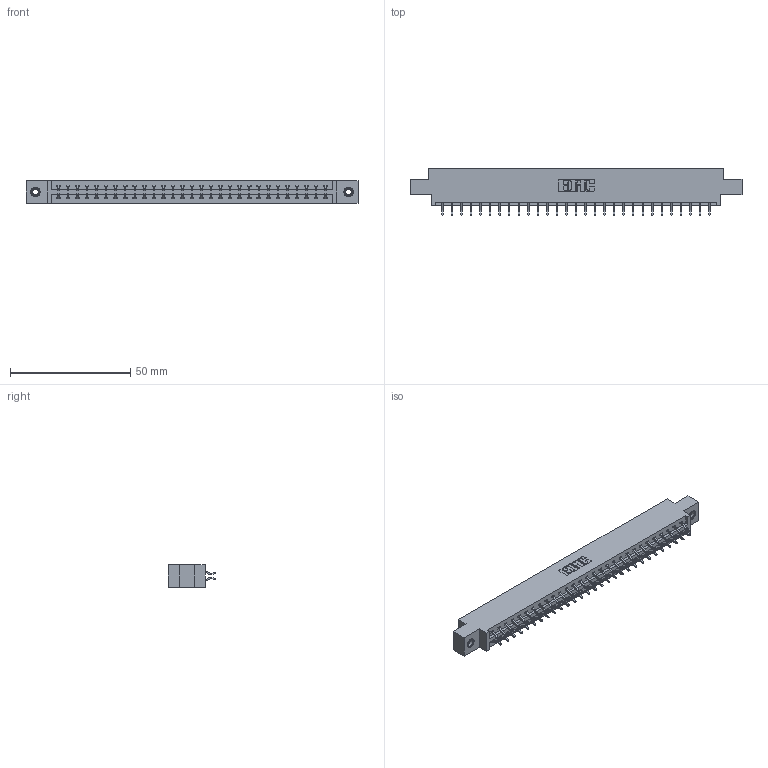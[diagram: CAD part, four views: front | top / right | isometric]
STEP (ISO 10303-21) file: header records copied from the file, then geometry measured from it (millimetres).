
FILE_DESCRIPTION (( 'STEP AP203' ), '1' );
FILE_NAME ('387-058-556-807.STEP', '2018-09-21T02:07:53', ( '' ), ( '' ), 'SwSTEP 2.0', 'SolidWorks 2016', '' );
FILE_SCHEMA (( 'CONFIG_CONTROL_DESIGN' ));
Length unit declared in the file: inch
Products named in the file (4): 345-292-001_556 Tail; 345-250-001_345-250-005-103; 387-058-556-807; 337 Part_0.170 Offset - 0.156 Dia-TI
Assembly tree (61 placements, depth 2):
  387-058-556-807
    337 Part_0.170 Offset - 0.156 Dia-TI
    345-292-001_556 Tail  x58
    345-250-001_345-250-005-103  x2
Bounding box: 137.92 x 19.57 x 9.4 mm (x, y, z)
Volume: 14229 mm3; surface area: 16042.2 mm2
Topology: 61 solids, 61 shells, 3658 faces, 10841 edges, 7142 vertices
Faces by surface type: plane 2542, cylinder 1100, cone 12, torus 4
Entity records: 25704 total; most frequent: CARTESIAN_POINT 4337, ORIENTED_EDGE 4254, DIRECTION 3733, EDGE_CURVE 2127, VECTOR 1971, LINE 1971, VERTEX_POINT 1412, AXIS2_PLACEMENT_3D 881
